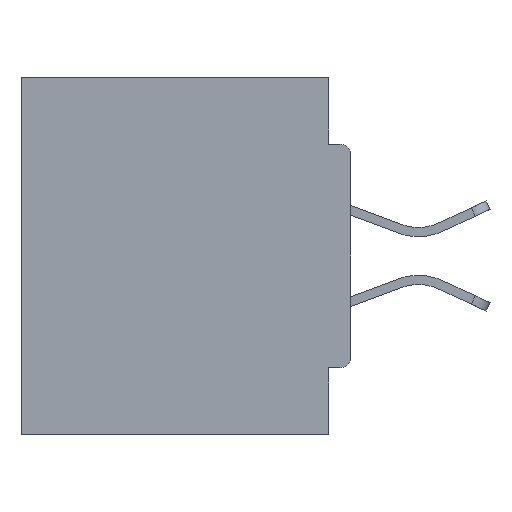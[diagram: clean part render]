
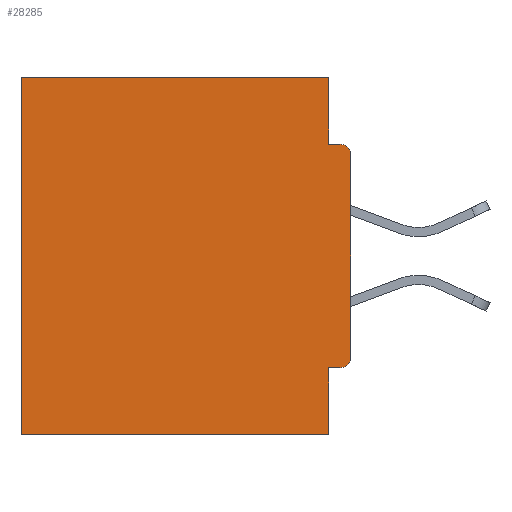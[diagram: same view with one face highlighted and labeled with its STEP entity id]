
A CAD part, left-side view. The second image highlights one B-rep face of the part: STEP entity #28285.
In plain terms, the highlighted planar face has unit normal (-1, 0, 0).
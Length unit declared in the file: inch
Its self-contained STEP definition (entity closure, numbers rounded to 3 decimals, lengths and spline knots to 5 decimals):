
#159 = ORIENTED_EDGE ( 'NONE', *, *, #34127, .F. ) ;
#318 = VERTEX_POINT ( 'NONE', #28804 ) ;
#692 = DIRECTION ( 'NONE',  ( 0., 1., 0. ) ) ;
#1042 = CARTESIAN_POINT ( 'NONE',  ( 0.298, 0.015, -0.0935 ) ) ;
#1350 = DIRECTION ( 'NONE',  ( 0., 1., 0. ) ) ;
#1524 = DIRECTION ( 'NONE',  ( 0., 1., 0. ) ) ;
#1908 = CARTESIAN_POINT ( 'NONE',  ( 0.298, 0., 0. ) ) ;
#2109 = DIRECTION ( 'NONE',  ( 0., 0., -1. ) ) ;
#2210 = LINE ( 'NONE', #4202, #17614 ) ;
#2887 = EDGE_CURVE ( 'NONE', #6937, #31933, #12028, .T. ) ;
#2932 = CARTESIAN_POINT ( 'NONE',  ( 0.298, 0., -0.3915 ) ) ;
#2986 = EDGE_CURVE ( 'NONE', #35187, #25579, #32485, .T. ) ;
#3611 = VECTOR ( 'NONE', #7628, 39.37008 ) ;
#3844 = AXIS2_PLACEMENT_3D ( 'NONE', #11362, #19994, #32408 ) ;
#4202 = CARTESIAN_POINT ( 'NONE',  ( 0.298, 0.031, -0.5 ) ) ;
#5166 = EDGE_LOOP ( 'NONE', ( #31297, #16634, #11171, #5358, #29562, #20329, #27344, #20625, #17690, #159 ) ) ;
#5358 = ORIENTED_EDGE ( 'NONE', *, *, #12830, .T. ) ;
#5437 = LINE ( 'NONE', #21248, #38611 ) ;
#5499 = VERTEX_POINT ( 'NONE', #24354 ) ;
#6823 = CARTESIAN_POINT ( 'NONE',  ( 0.298, 0.46, -0.5 ) ) ;
#6937 = VERTEX_POINT ( 'NONE', #15807 ) ;
#7628 = DIRECTION ( 'NONE',  ( 0., 0., -1. ) ) ;
#8112 = VECTOR ( 'NONE', #13951, 39.37008 ) ;
#8454 = LINE ( 'NONE', #19945, #15013 ) ;
#8935 = DIRECTION ( 'NONE',  ( 0., 0., -1. ) ) ;
#9312 = CARTESIAN_POINT ( 'NONE',  ( 0.298, 0.031, -0.4065 ) ) ;
#11171 = ORIENTED_EDGE ( 'NONE', *, *, #2887, .F. ) ;
#11362 = CARTESIAN_POINT ( 'NONE',  ( 0.298, 0.015, -0.3915 ) ) ;
#12028 = LINE ( 'NONE', #21848, #34924 ) ;
#12830 = EDGE_CURVE ( 'NONE', #6937, #318, #5437, .T. ) ;
#13343 = CARTESIAN_POINT ( 'NONE',  ( 0.298, 0., -0.4065 ) ) ;
#13373 = EDGE_CURVE ( 'NONE', #5499, #16144, #35288, .T. ) ;
#13742 = PLANE ( 'NONE',  #14117 ) ;
#13786 = LINE ( 'NONE', #22125, #3611 ) ;
#13820 = CARTESIAN_POINT ( 'NONE',  ( 0.298, 0., -0.0935 ) ) ;
#13951 = DIRECTION ( 'NONE',  ( 0., -1., 0. ) ) ;
#14117 = AXIS2_PLACEMENT_3D ( 'NONE', #1908, #23248, #8935 ) ;
#14634 = EDGE_CURVE ( 'NONE', #35187, #38506, #34241, .T. ) ;
#15013 = VECTOR ( 'NONE', #2109, 39.37008 ) ;
#15205 = LINE ( 'NONE', #37755, #38576 ) ;
#15807 = CARTESIAN_POINT ( 'NONE',  ( 0.298, 0.031, 0. ) ) ;
#16144 = VERTEX_POINT ( 'NONE', #1042 ) ;
#16634 = ORIENTED_EDGE ( 'NONE', *, *, #20744, .F. ) ;
#17614 = VECTOR ( 'NONE', #31573, 39.37008 ) ;
#17690 = ORIENTED_EDGE ( 'NONE', *, *, #14634, .T. ) ;
#18152 = VERTEX_POINT ( 'NONE', #35501 ) ;
#19945 = CARTESIAN_POINT ( 'NONE',  ( 0.298, 0.46, 0. ) ) ;
#19994 = DIRECTION ( 'NONE',  ( -1., 0., 0. ) ) ;
#20329 = ORIENTED_EDGE ( 'NONE', *, *, #36441, .F. ) ;
#20625 = ORIENTED_EDGE ( 'NONE', *, *, #2986, .F. ) ;
#20744 = EDGE_CURVE ( 'NONE', #31933, #16144, #23524, .T. ) ;
#21248 = CARTESIAN_POINT ( 'NONE',  ( 0.298, 0., 0. ) ) ;
#21848 = CARTESIAN_POINT ( 'NONE',  ( 0.298, 0.031, -0.5 ) ) ;
#22125 = CARTESIAN_POINT ( 'NONE',  ( 0.298, 0., 0. ) ) ;
#23120 = VERTEX_POINT ( 'NONE', #6823 ) ;
#23248 = DIRECTION ( 'NONE',  ( 1., 0., 0. ) ) ;
#23343 = DIRECTION ( 'NONE',  ( 0., 0., -1. ) ) ;
#23524 = LINE ( 'NONE', #13820, #8112 ) ;
#23735 = DIRECTION ( 'NONE',  ( -1., 0., 0. ) ) ;
#24354 = CARTESIAN_POINT ( 'NONE',  ( 0.298, 0., -0.1085 ) ) ;
#24749 = AXIS2_PLACEMENT_3D ( 'NONE', #26616, #23735, #23343 ) ;
#25579 = VERTEX_POINT ( 'NONE', #9312 ) ;
#26616 = CARTESIAN_POINT ( 'NONE',  ( 0.298, 0.015, -0.1085 ) ) ;
#27293 = VECTOR ( 'NONE', #1524, 39.37008 ) ;
#27344 = ORIENTED_EDGE ( 'NONE', *, *, #35337, .F. ) ;
#28070 = CARTESIAN_POINT ( 'NONE',  ( 0.298, 0.031, -0.0935 ) ) ;
#28256 = DIRECTION ( 'NONE',  ( 0., 0., -1. ) ) ;
#28285 = ADVANCED_FACE ( 'NONE', ( #36268 ), #13742, .F. ) ;
#28804 = CARTESIAN_POINT ( 'NONE',  ( 0.298, 0.46, 0. ) ) ;
#29562 = ORIENTED_EDGE ( 'NONE', *, *, #33790, .T. ) ;
#31297 = ORIENTED_EDGE ( 'NONE', *, *, #13373, .T. ) ;
#31573 = DIRECTION ( 'NONE',  ( 0., 0., -1. ) ) ;
#31933 = VERTEX_POINT ( 'NONE', #28070 ) ;
#32408 = DIRECTION ( 'NONE',  ( 0., 0., -1. ) ) ;
#32485 = LINE ( 'NONE', #13343, #27293 ) ;
#33790 = EDGE_CURVE ( 'NONE', #318, #23120, #8454, .T. ) ;
#34127 = EDGE_CURVE ( 'NONE', #5499, #38506, #13786, .T. ) ;
#34241 = CIRCLE ( 'NONE', #3844, 0.015 ) ;
#34924 = VECTOR ( 'NONE', #28256, 39.37008 ) ;
#35187 = VERTEX_POINT ( 'NONE', #36902 ) ;
#35288 = CIRCLE ( 'NONE', #24749, 0.015 ) ;
#35337 = EDGE_CURVE ( 'NONE', #25579, #18152, #2210, .T. ) ;
#35501 = CARTESIAN_POINT ( 'NONE',  ( 0.298, 0.031, -0.5 ) ) ;
#36268 = FACE_OUTER_BOUND ( 'NONE', #5166, .T. ) ;
#36441 = EDGE_CURVE ( 'NONE', #18152, #23120, #15205, .T. ) ;
#36902 = CARTESIAN_POINT ( 'NONE',  ( 0.298, 0.015, -0.4065 ) ) ;
#37755 = CARTESIAN_POINT ( 'NONE',  ( 0.298, 0., -0.5 ) ) ;
#38506 = VERTEX_POINT ( 'NONE', #2932 ) ;
#38576 = VECTOR ( 'NONE', #1350, 39.37008 ) ;
#38611 = VECTOR ( 'NONE', #692, 39.37008 ) ;
